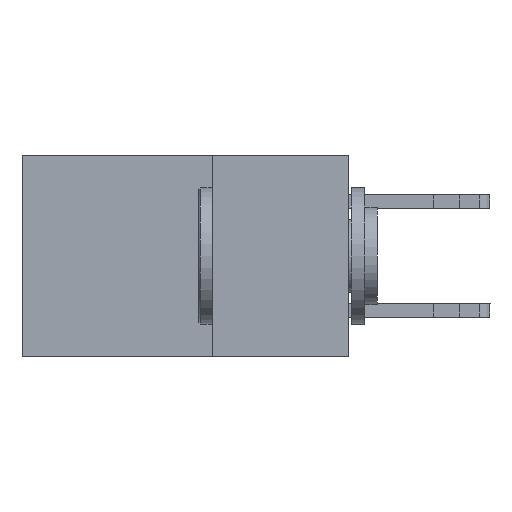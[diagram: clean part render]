
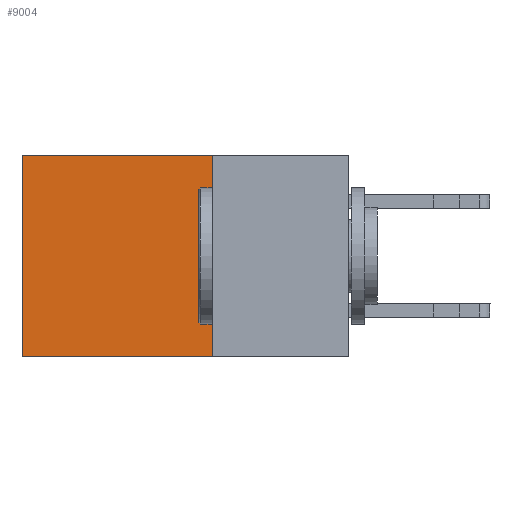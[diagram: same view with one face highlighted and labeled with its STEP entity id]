
A CAD part, left-side view. The second image highlights one B-rep face of the part: STEP entity #9004.
In plain terms, the highlighted planar face has unit normal (-1, 0, 0).
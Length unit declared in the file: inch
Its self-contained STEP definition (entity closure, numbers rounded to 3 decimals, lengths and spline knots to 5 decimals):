
#974 = CARTESIAN_POINT ( 'NONE',  ( 0.298, 0.25, -0.37 ) ) ;
#1398 = CARTESIAN_POINT ( 'NONE',  ( 0.298, 0.25, 0. ) ) ;
#1708 = VERTEX_POINT ( 'NONE', #1398 ) ;
#1982 = VECTOR ( 'NONE', #3929, 39.37008 ) ;
#2149 = LINE ( 'NONE', #2303, #17554 ) ;
#2276 = LINE ( 'NONE', #10213, #17461 ) ;
#2303 = CARTESIAN_POINT ( 'NONE',  ( 0.298, 0.25, 0. ) ) ;
#2466 = EDGE_CURVE ( 'NONE', #1708, #10412, #2149, .T. ) ;
#2604 = DIRECTION ( 'NONE',  ( 0., 0., -1. ) ) ;
#2824 = LINE ( 'NONE', #974, #1982 ) ;
#3595 = VECTOR ( 'NONE', #6256, 39.37008 ) ;
#3712 = FACE_OUTER_BOUND ( 'NONE', #4013, .T. ) ;
#3871 = DIRECTION ( 'NONE',  ( 1., 0., 0. ) ) ;
#3908 = CARTESIAN_POINT ( 'NONE',  ( 0.298, 0.25, -0.37 ) ) ;
#3929 = DIRECTION ( 'NONE',  ( 0., 1., 0. ) ) ;
#4013 = EDGE_LOOP ( 'NONE', ( #11885, #16731, #14485, #9356 ) ) ;
#4834 = DIRECTION ( 'NONE',  ( 0., 1., 0. ) ) ;
#6256 = DIRECTION ( 'NONE',  ( 0., 0., -1. ) ) ;
#8699 = VERTEX_POINT ( 'NONE', #16679 ) ;
#9004 = ADVANCED_FACE ( 'NONE', ( #3712 ), #12114, .F. ) ;
#9115 = DIRECTION ( 'NONE',  ( 0., 0., -1. ) ) ;
#9198 = VERTEX_POINT ( 'NONE', #3908 ) ;
#9206 = CARTESIAN_POINT ( 'NONE',  ( 0.298, 0.6, 0. ) ) ;
#9335 = CARTESIAN_POINT ( 'NONE',  ( 0.298, 0.25, 0. ) ) ;
#9356 = ORIENTED_EDGE ( 'NONE', *, *, #2466, .T. ) ;
#10191 = CARTESIAN_POINT ( 'NONE',  ( 0.298, 0.25, 0. ) ) ;
#10213 = CARTESIAN_POINT ( 'NONE',  ( 0.298, 0.6, 0. ) ) ;
#10412 = VERTEX_POINT ( 'NONE', #9206 ) ;
#10609 = EDGE_CURVE ( 'NONE', #9198, #8699, #2824, .T. ) ;
#11885 = ORIENTED_EDGE ( 'NONE', *, *, #15269, .T. ) ;
#12114 = PLANE ( 'NONE',  #13261 ) ;
#12374 = LINE ( 'NONE', #10191, #3595 ) ;
#13261 = AXIS2_PLACEMENT_3D ( 'NONE', #9335, #3871, #2604 ) ;
#14413 = EDGE_CURVE ( 'NONE', #1708, #9198, #12374, .T. ) ;
#14485 = ORIENTED_EDGE ( 'NONE', *, *, #14413, .F. ) ;
#15269 = EDGE_CURVE ( 'NONE', #10412, #8699, #2276, .T. ) ;
#16679 = CARTESIAN_POINT ( 'NONE',  ( 0.298, 0.6, -0.37 ) ) ;
#16731 = ORIENTED_EDGE ( 'NONE', *, *, #10609, .F. ) ;
#17461 = VECTOR ( 'NONE', #9115, 39.37008 ) ;
#17554 = VECTOR ( 'NONE', #4834, 39.37008 ) ;
